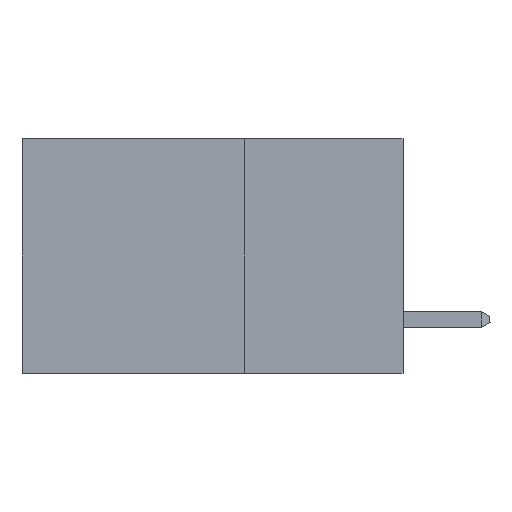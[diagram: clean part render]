
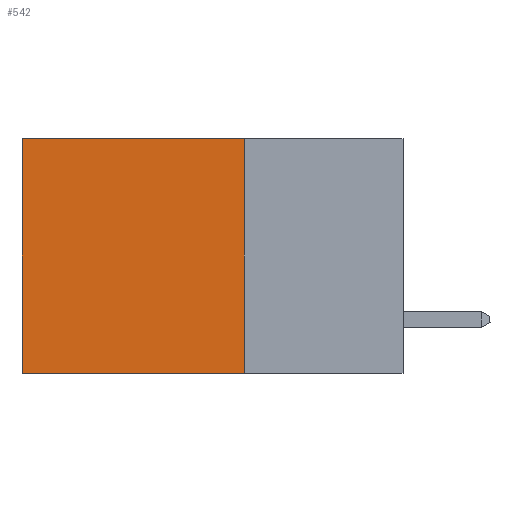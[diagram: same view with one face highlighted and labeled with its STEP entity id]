
A CAD part, left-side view. The second image highlights one B-rep face of the part: STEP entity #542.
In plain terms, the highlighted planar face has unit normal (-1, 0, 0).
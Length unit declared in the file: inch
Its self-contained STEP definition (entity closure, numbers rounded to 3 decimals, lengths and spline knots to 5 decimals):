
#65 = EDGE_LOOP ( 'NONE', ( #4749, #3620, #9359, #8588 ) ) ;
#260 = AXIS2_PLACEMENT_3D ( 'NONE', #7110, #2177, #10377 ) ;
#542 = ADVANCED_FACE ( 'NONE', ( #4082 ), #6219, .F. ) ;
#978 = CARTESIAN_POINT ( 'NONE',  ( 0.2875, 0.25, -0.37 ) ) ;
#1728 = DIRECTION ( 'NONE',  ( 0., 1., 0. ) ) ;
#1855 = VECTOR ( 'NONE', #8461, 39.37008 ) ;
#2177 = DIRECTION ( 'NONE',  ( 1., 0., 0. ) ) ;
#3227 = DIRECTION ( 'NONE',  ( 0., 0., -1. ) ) ;
#3349 = CARTESIAN_POINT ( 'NONE',  ( 0.2875, 0.25, 0. ) ) ;
#3490 = EDGE_CURVE ( 'NONE', #10132, #8406, #4531, .T. ) ;
#3571 = VERTEX_POINT ( 'NONE', #3799 ) ;
#3620 = ORIENTED_EDGE ( 'NONE', *, *, #8407, .F. ) ;
#3799 = CARTESIAN_POINT ( 'NONE',  ( 0.2875, 0.6, -0.37 ) ) ;
#4082 = FACE_OUTER_BOUND ( 'NONE', #65, .T. ) ;
#4531 = LINE ( 'NONE', #7727, #1855 ) ;
#4749 = ORIENTED_EDGE ( 'NONE', *, *, #7671, .T. ) ;
#4808 = CARTESIAN_POINT ( 'NONE',  ( 0.2875, 0.6, 0. ) ) ;
#5831 = LINE ( 'NONE', #4808, #9698 ) ;
#6219 = PLANE ( 'NONE',  #260 ) ;
#6640 = VECTOR ( 'NONE', #9073, 39.37008 ) ;
#7110 = CARTESIAN_POINT ( 'NONE',  ( 0.2875, 0.25, 0. ) ) ;
#7186 = VECTOR ( 'NONE', #1728, 39.37008 ) ;
#7671 = EDGE_CURVE ( 'NONE', #8500, #3571, #5831, .T. ) ;
#7727 = CARTESIAN_POINT ( 'NONE',  ( 0.2875, 0.25, 0. ) ) ;
#7916 = CARTESIAN_POINT ( 'NONE',  ( 0.2875, 0.25, 0. ) ) ;
#8406 = VERTEX_POINT ( 'NONE', #9120 ) ;
#8407 = EDGE_CURVE ( 'NONE', #8406, #3571, #9920, .T. ) ;
#8461 = DIRECTION ( 'NONE',  ( 0., 0., -1. ) ) ;
#8500 = VERTEX_POINT ( 'NONE', #10124 ) ;
#8588 = ORIENTED_EDGE ( 'NONE', *, *, #9701, .T. ) ;
#9073 = DIRECTION ( 'NONE',  ( 0., 1., 0. ) ) ;
#9120 = CARTESIAN_POINT ( 'NONE',  ( 0.2875, 0.25, -0.37 ) ) ;
#9359 = ORIENTED_EDGE ( 'NONE', *, *, #3490, .F. ) ;
#9698 = VECTOR ( 'NONE', #3227, 39.37008 ) ;
#9701 = EDGE_CURVE ( 'NONE', #10132, #8500, #10540, .T. ) ;
#9920 = LINE ( 'NONE', #978, #7186 ) ;
#10124 = CARTESIAN_POINT ( 'NONE',  ( 0.2875, 0.6, 0. ) ) ;
#10132 = VERTEX_POINT ( 'NONE', #7916 ) ;
#10377 = DIRECTION ( 'NONE',  ( 0., 0., -1. ) ) ;
#10540 = LINE ( 'NONE', #3349, #6640 ) ;
